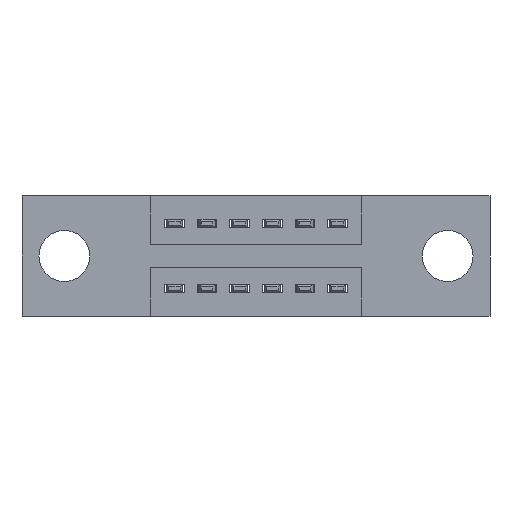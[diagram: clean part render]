
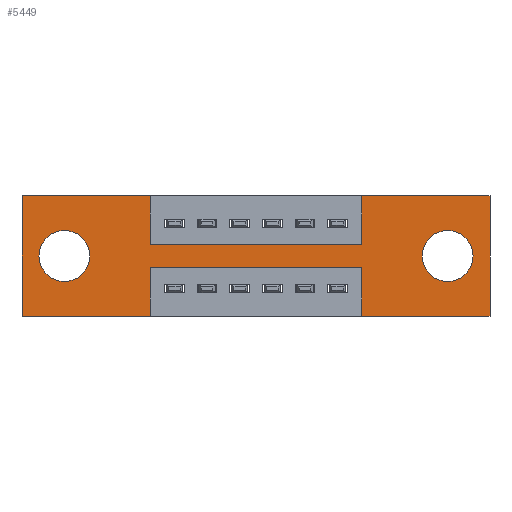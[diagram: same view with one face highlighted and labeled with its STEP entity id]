
A CAD part, front view. The second image highlights one B-rep face of the part: STEP entity #5449.
In plain terms, the highlighted planar face has unit normal (0, -1, 0).
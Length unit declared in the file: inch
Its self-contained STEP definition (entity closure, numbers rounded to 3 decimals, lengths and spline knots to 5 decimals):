
#17 = VERTEX_POINT ( 'NONE', #4791 ) ;
#148 = VERTEX_POINT ( 'NONE', #2747 ) ;
#247 = AXIS2_PLACEMENT_3D ( 'NONE', #5436, #8990, #6727 ) ;
#249 = DIRECTION ( 'NONE',  ( 1., 0., 0. ) ) ;
#287 = CARTESIAN_POINT ( 'NONE',  ( 1.305, 0., -0.263 ) ) ;
#326 = LINE ( 'NONE', #542, #7865 ) ;
#333 = CARTESIAN_POINT ( 'NONE',  ( 1.435, 0., -0.37 ) ) ;
#482 = VECTOR ( 'NONE', #9360, 39.37008 ) ;
#484 = DIRECTION ( 'NONE',  ( -1., 0., 0. ) ) ;
#542 = CARTESIAN_POINT ( 'NONE',  ( 0.3925, 0., 0. ) ) ;
#583 = CIRCLE ( 'NONE', #7100, 0.078 ) ;
#610 = DIRECTION ( 'NONE',  ( 0., 1., 0. ) ) ;
#637 = DIRECTION ( 'NONE',  ( 0., 0., -1. ) ) ;
#729 = LINE ( 'NONE', #3476, #8181 ) ;
#744 = CIRCLE ( 'NONE', #1970, 0.078 ) ;
#805 = ORIENTED_EDGE ( 'NONE', *, *, #2194, .F. ) ;
#875 = VERTEX_POINT ( 'NONE', #6320 ) ;
#881 = VECTOR ( 'NONE', #3087, 39.37008 ) ;
#924 = FACE_OUTER_BOUND ( 'NONE', #5464, .T. ) ;
#1016 = VECTOR ( 'NONE', #1295, 39.37008 ) ;
#1140 = CARTESIAN_POINT ( 'NONE',  ( 1.0425, 0., -0.37 ) ) ;
#1148 = EDGE_CURVE ( 'NONE', #2213, #3827, #2027, .T. ) ;
#1282 = EDGE_CURVE ( 'NONE', #2539, #2494, #5261, .T. ) ;
#1295 = DIRECTION ( 'NONE',  ( -1., 0., 0. ) ) ;
#1522 = DIRECTION ( 'NONE',  ( 0., 0., 1. ) ) ;
#1602 = AXIS2_PLACEMENT_3D ( 'NONE', #2743, #2657, #2655 ) ;
#1645 = EDGE_CURVE ( 'NONE', #8642, #7427, #3001, .T. ) ;
#1720 = VECTOR ( 'NONE', #5729, 39.37008 ) ;
#1770 = ORIENTED_EDGE ( 'NONE', *, *, #1877, .F. ) ;
#1800 = EDGE_CURVE ( 'NONE', #148, #1977, #5468, .T. ) ;
#1826 = ORIENTED_EDGE ( 'NONE', *, *, #1148, .F. ) ;
#1841 = EDGE_CURVE ( 'NONE', #6681, #2824, #744, .T. ) ;
#1877 = EDGE_CURVE ( 'NONE', #17, #8642, #6723, .T. ) ;
#1908 = EDGE_CURVE ( 'NONE', #9201, #17, #3958, .T. ) ;
#1934 = EDGE_CURVE ( 'NONE', #2494, #9201, #7572, .T. ) ;
#1970 = AXIS2_PLACEMENT_3D ( 'NONE', #6708, #7196, #7174 ) ;
#1977 = VERTEX_POINT ( 'NONE', #287 ) ;
#2027 = LINE ( 'NONE', #2871, #5881 ) ;
#2149 = VECTOR ( 'NONE', #484, 39.37008 ) ;
#2194 = EDGE_CURVE ( 'NONE', #3045, #2805, #3109, .T. ) ;
#2210 = EDGE_CURVE ( 'NONE', #875, #3045, #729, .T. ) ;
#2213 = VERTEX_POINT ( 'NONE', #4702 ) ;
#2403 = CARTESIAN_POINT ( 'NONE',  ( 1.435, 0., 0. ) ) ;
#2407 = VECTOR ( 'NONE', #637, 39.37008 ) ;
#2494 = VERTEX_POINT ( 'NONE', #1140 ) ;
#2539 = VERTEX_POINT ( 'NONE', #333 ) ;
#2583 = EDGE_CURVE ( 'NONE', #3827, #875, #326, .T. ) ;
#2655 = DIRECTION ( 'NONE',  ( 0., 0., -1. ) ) ;
#2657 = DIRECTION ( 'NONE',  ( 0., -1., 0. ) ) ;
#2658 = ORIENTED_EDGE ( 'NONE', *, *, #3623, .T. ) ;
#2684 = ORIENTED_EDGE ( 'NONE', *, *, #2748, .F. ) ;
#2743 = CARTESIAN_POINT ( 'NONE',  ( 0., 0., -0.37 ) ) ;
#2747 = CARTESIAN_POINT ( 'NONE',  ( 1.305, 0., -0.107 ) ) ;
#2748 = EDGE_CURVE ( 'NONE', #2805, #8999, #7458, .T. ) ;
#2754 = PLANE ( 'NONE',  #1602 ) ;
#2801 = FACE_BOUND ( 'NONE', #8769, .T. ) ;
#2805 = VERTEX_POINT ( 'NONE', #7593 ) ;
#2824 = VERTEX_POINT ( 'NONE', #6394 ) ;
#2860 = DIRECTION ( 'NONE',  ( 0., 0., 1. ) ) ;
#2871 = CARTESIAN_POINT ( 'NONE',  ( 0., 0., 0. ) ) ;
#3001 = LINE ( 'NONE', #8745, #881 ) ;
#3045 = VERTEX_POINT ( 'NONE', #6863 ) ;
#3087 = DIRECTION ( 'NONE',  ( -1., 0., 0. ) ) ;
#3109 = LINE ( 'NONE', #3385, #5019 ) ;
#3115 = EDGE_CURVE ( 'NONE', #2824, #6681, #583, .T. ) ;
#3162 = ORIENTED_EDGE ( 'NONE', *, *, #2210, .F. ) ;
#3385 = CARTESIAN_POINT ( 'NONE',  ( 1.0425, 0., 0. ) ) ;
#3476 = CARTESIAN_POINT ( 'NONE',  ( 0.3925, 0., -0.15 ) ) ;
#3623 = EDGE_CURVE ( 'NONE', #1977, #148, #4079, .T. ) ;
#3679 = CARTESIAN_POINT ( 'NONE',  ( 0.3925, 0., -0.37 ) ) ;
#3743 = ORIENTED_EDGE ( 'NONE', *, *, #7063, .F. ) ;
#3790 = ORIENTED_EDGE ( 'NONE', *, *, #1800, .T. ) ;
#3827 = VERTEX_POINT ( 'NONE', #9187 ) ;
#3863 = VECTOR ( 'NONE', #6140, 39.37008 ) ;
#3958 = LINE ( 'NONE', #8564, #2149 ) ;
#3998 = ORIENTED_EDGE ( 'NONE', *, *, #1908, .F. ) ;
#4079 = CIRCLE ( 'NONE', #247, 0.078 ) ;
#4258 = ORIENTED_EDGE ( 'NONE', *, *, #1645, .F. ) ;
#4280 = ORIENTED_EDGE ( 'NONE', *, *, #1934, .F. ) ;
#4406 = CARTESIAN_POINT ( 'NONE',  ( 1.435, 0., 0. ) ) ;
#4468 = ORIENTED_EDGE ( 'NONE', *, *, #5890, .F. ) ;
#4604 = CARTESIAN_POINT ( 'NONE',  ( 0., 0., 0. ) ) ;
#4702 = CARTESIAN_POINT ( 'NONE',  ( 0., 0., 0. ) ) ;
#4778 = LINE ( 'NONE', #2403, #482 ) ;
#4791 = CARTESIAN_POINT ( 'NONE',  ( 0.3925, 0., -0.22 ) ) ;
#4946 = FACE_BOUND ( 'NONE', #6082, .T. ) ;
#5019 = VECTOR ( 'NONE', #5366, 39.37008 ) ;
#5201 = CARTESIAN_POINT ( 'NONE',  ( 0., 0., -0.37 ) ) ;
#5261 = LINE ( 'NONE', #5901, #1016 ) ;
#5366 = DIRECTION ( 'NONE',  ( 0., 0., 1. ) ) ;
#5373 = DIRECTION ( 'NONE',  ( 1., 0., 0. ) ) ;
#5387 = DIRECTION ( 'NONE',  ( 0., 0., -1. ) ) ;
#5436 = CARTESIAN_POINT ( 'NONE',  ( 1.305, 0., -0.185 ) ) ;
#5449 = ADVANCED_FACE ( 'NONE', ( #4946, #2801, #924 ), #2754, .T. ) ;
#5462 = CARTESIAN_POINT ( 'NONE',  ( 1.305, 0., -0.185 ) ) ;
#5464 = EDGE_LOOP ( 'NONE', ( #1770, #3998, #4280, #6261, #3743, #2684, #805, #3162, #8686, #1826, #4468, #4258 ) ) ;
#5468 = CIRCLE ( 'NONE', #9241, 0.078 ) ;
#5556 = VECTOR ( 'NONE', #2860, 39.37008 ) ;
#5692 = ORIENTED_EDGE ( 'NONE', *, *, #3115, .T. ) ;
#5729 = DIRECTION ( 'NONE',  ( 1., 0., 0. ) ) ;
#5881 = VECTOR ( 'NONE', #249, 39.37008 ) ;
#5890 = EDGE_CURVE ( 'NONE', #7427, #2213, #9319, .T. ) ;
#5901 = CARTESIAN_POINT ( 'NONE',  ( 0., 0., -0.37 ) ) ;
#6082 = EDGE_LOOP ( 'NONE', ( #3790, #2658 ) ) ;
#6140 = DIRECTION ( 'NONE',  ( 0., 0., 1. ) ) ;
#6261 = ORIENTED_EDGE ( 'NONE', *, *, #1282, .F. ) ;
#6320 = CARTESIAN_POINT ( 'NONE',  ( 0.3925, 0., -0.15 ) ) ;
#6394 = CARTESIAN_POINT ( 'NONE',  ( 0.13, 0., -0.263 ) ) ;
#6459 = CARTESIAN_POINT ( 'NONE',  ( 0., 0., 0. ) ) ;
#6561 = ORIENTED_EDGE ( 'NONE', *, *, #1841, .T. ) ;
#6681 = VERTEX_POINT ( 'NONE', #9100 ) ;
#6708 = CARTESIAN_POINT ( 'NONE',  ( 0.13, 0., -0.185 ) ) ;
#6723 = LINE ( 'NONE', #3679, #2407 ) ;
#6727 = DIRECTION ( 'NONE',  ( 0., 0., -1. ) ) ;
#6863 = CARTESIAN_POINT ( 'NONE',  ( 1.0425, 0., -0.15 ) ) ;
#6974 = DIRECTION ( 'NONE',  ( 0., 1., 0. ) ) ;
#7063 = EDGE_CURVE ( 'NONE', #8999, #2539, #4778, .T. ) ;
#7100 = AXIS2_PLACEMENT_3D ( 'NONE', #7939, #6974, #1522 ) ;
#7159 = CARTESIAN_POINT ( 'NONE',  ( 1.0425, 0., -0.37 ) ) ;
#7174 = DIRECTION ( 'NONE',  ( 0., 0., 1. ) ) ;
#7196 = DIRECTION ( 'NONE',  ( 0., 1., 0. ) ) ;
#7427 = VERTEX_POINT ( 'NONE', #5201 ) ;
#7458 = LINE ( 'NONE', #4604, #1720 ) ;
#7572 = LINE ( 'NONE', #7159, #5556 ) ;
#7593 = CARTESIAN_POINT ( 'NONE',  ( 1.0425, 0., 0. ) ) ;
#7865 = VECTOR ( 'NONE', #9116, 39.37008 ) ;
#7939 = CARTESIAN_POINT ( 'NONE',  ( 0.13, 0., -0.185 ) ) ;
#8050 = CARTESIAN_POINT ( 'NONE',  ( 0.3925, 0., -0.37 ) ) ;
#8181 = VECTOR ( 'NONE', #5373, 39.37008 ) ;
#8490 = CARTESIAN_POINT ( 'NONE',  ( 1.0425, 0., -0.22 ) ) ;
#8564 = CARTESIAN_POINT ( 'NONE',  ( 0.3925, 0., -0.22 ) ) ;
#8642 = VERTEX_POINT ( 'NONE', #8050 ) ;
#8686 = ORIENTED_EDGE ( 'NONE', *, *, #2583, .F. ) ;
#8745 = CARTESIAN_POINT ( 'NONE',  ( 0., 0., -0.37 ) ) ;
#8769 = EDGE_LOOP ( 'NONE', ( #6561, #5692 ) ) ;
#8990 = DIRECTION ( 'NONE',  ( 0., 1., 0. ) ) ;
#8999 = VERTEX_POINT ( 'NONE', #4406 ) ;
#9100 = CARTESIAN_POINT ( 'NONE',  ( 0.13, 0., -0.107 ) ) ;
#9116 = DIRECTION ( 'NONE',  ( 0., 0., -1. ) ) ;
#9187 = CARTESIAN_POINT ( 'NONE',  ( 0.3925, 0., 0. ) ) ;
#9201 = VERTEX_POINT ( 'NONE', #8490 ) ;
#9241 = AXIS2_PLACEMENT_3D ( 'NONE', #5462, #610, #5387 ) ;
#9319 = LINE ( 'NONE', #6459, #3863 ) ;
#9360 = DIRECTION ( 'NONE',  ( 0., 0., -1. ) ) ;
